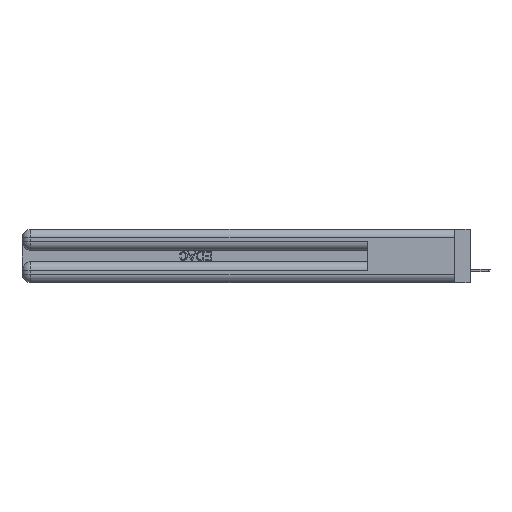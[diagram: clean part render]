
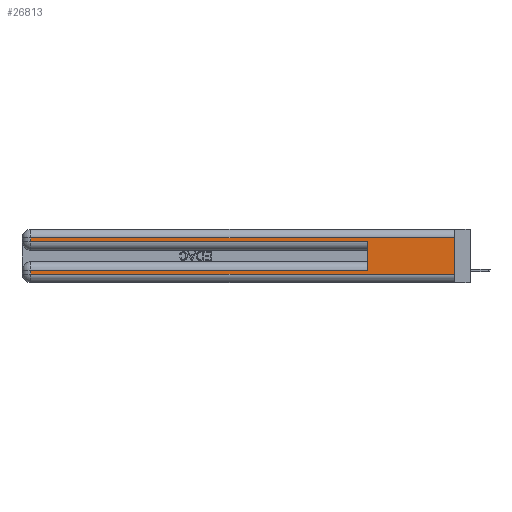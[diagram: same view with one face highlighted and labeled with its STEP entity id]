
A CAD part, left-side view. The second image highlights one B-rep face of the part: STEP entity #26813.
In plain terms, the highlighted planar face has unit normal (-1, 0, 0).
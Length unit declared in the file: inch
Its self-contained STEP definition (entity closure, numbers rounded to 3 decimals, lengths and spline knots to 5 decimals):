
#899 = DIRECTION ( 'NONE',  ( 0., 0., 1. ) ) ;
#1643 = EDGE_CURVE ( 'NONE', #45693, #24644, #16092, .T. ) ;
#1722 = CARTESIAN_POINT ( 'NONE',  ( 0., 0., 0.37 ) ) ;
#3367 = VECTOR ( 'NONE', #18326, 39.37008 ) ;
#3854 = VERTEX_POINT ( 'NONE', #38663 ) ;
#4175 = VECTOR ( 'NONE', #27607, 39.37008 ) ;
#5422 = CARTESIAN_POINT ( 'NONE',  ( 0., 0.6, 0.085 ) ) ;
#5464 = LINE ( 'NONE', #36732, #3367 ) ;
#6622 = ORIENTED_EDGE ( 'NONE', *, *, #1643, .T. ) ;
#7511 = EDGE_CURVE ( 'NONE', #30257, #46423, #32999, .T. ) ;
#7593 = CARTESIAN_POINT ( 'NONE',  ( 0., 0., 0.085 ) ) ;
#7675 = VECTOR ( 'NONE', #27353, 39.37008 ) ;
#7863 = VECTOR ( 'NONE', #13284, 39.37008 ) ;
#7893 = DIRECTION ( 'NONE',  ( 0., -1., 0. ) ) ;
#9753 = ORIENTED_EDGE ( 'NONE', *, *, #15042, .T. ) ;
#11579 = EDGE_CURVE ( 'NONE', #45693, #19201, #28604, .T. ) ;
#12773 = EDGE_LOOP ( 'NONE', ( #22890, #43715, #9753, #49290, #46604, #6622, #43166, #16852 ) ) ;
#13091 = CARTESIAN_POINT ( 'NONE',  ( 0., 0., 0.06 ) ) ;
#13197 = CARTESIAN_POINT ( 'NONE',  ( 0., 2.94, 0.37 ) ) ;
#13284 = DIRECTION ( 'NONE',  ( 0., 0., -1. ) ) ;
#13481 = VERTEX_POINT ( 'NONE', #21888 ) ;
#15042 = EDGE_CURVE ( 'NONE', #24891, #3854, #47481, .T. ) ;
#15576 = LINE ( 'NONE', #31188, #7675 ) ;
#16092 = LINE ( 'NONE', #7593, #4175 ) ;
#16577 = DIRECTION ( 'NONE',  ( 0., 0., -1. ) ) ;
#16852 = ORIENTED_EDGE ( 'NONE', *, *, #35862, .T. ) ;
#18326 = DIRECTION ( 'NONE',  ( 0., 0., -1. ) ) ;
#19201 = VERTEX_POINT ( 'NONE', #46663 ) ;
#19489 = CARTESIAN_POINT ( 'NONE',  ( 0., 0., 0.06 ) ) ;
#19550 = VECTOR ( 'NONE', #899, 39.37008 ) ;
#21888 = CARTESIAN_POINT ( 'NONE',  ( 0., 2.94, 0.06 ) ) ;
#22890 = ORIENTED_EDGE ( 'NONE', *, *, #7511, .F. ) ;
#23029 = EDGE_CURVE ( 'NONE', #3854, #19201, #50371, .T. ) ;
#24139 = DIRECTION ( 'NONE',  ( 0., -1., 0. ) ) ;
#24644 = VERTEX_POINT ( 'NONE', #34574 ) ;
#24891 = VERTEX_POINT ( 'NONE', #37285 ) ;
#26459 = DIRECTION ( 'NONE',  ( 1., 0., 0. ) ) ;
#26609 = EDGE_CURVE ( 'NONE', #30257, #24891, #15576, .T. ) ;
#26702 = CARTESIAN_POINT ( 'NONE',  ( 0., 0., 0.37 ) ) ;
#26813 = ADVANCED_FACE ( 'NONE', ( #30568 ), #42778, .F. ) ;
#26869 = CARTESIAN_POINT ( 'NONE',  ( 0., 0., 0.285 ) ) ;
#27353 = DIRECTION ( 'NONE',  ( 0., 1., 0. ) ) ;
#27607 = DIRECTION ( 'NONE',  ( 0., 1., 0. ) ) ;
#28088 = VECTOR ( 'NONE', #24139, 39.37008 ) ;
#28604 = LINE ( 'NONE', #36000, #19550 ) ;
#30257 = VERTEX_POINT ( 'NONE', #45720 ) ;
#30568 = FACE_OUTER_BOUND ( 'NONE', #12773, .T. ) ;
#31188 = CARTESIAN_POINT ( 'NONE',  ( 0., 0., 0.31 ) ) ;
#32999 = LINE ( 'NONE', #1722, #7863 ) ;
#34262 = EDGE_CURVE ( 'NONE', #24644, #13481, #5464, .T. ) ;
#34574 = CARTESIAN_POINT ( 'NONE',  ( 0., 2.94, 0.085 ) ) ;
#35625 = LINE ( 'NONE', #13091, #28088 ) ;
#35862 = EDGE_CURVE ( 'NONE', #13481, #46423, #35625, .T. ) ;
#36000 = CARTESIAN_POINT ( 'NONE',  ( 0., 0.6, 0.145 ) ) ;
#36316 = AXIS2_PLACEMENT_3D ( 'NONE', #26702, #26459, #50455 ) ;
#36732 = CARTESIAN_POINT ( 'NONE',  ( 0., 2.94, 0.37 ) ) ;
#37285 = CARTESIAN_POINT ( 'NONE',  ( 0., 2.94, 0.31 ) ) ;
#38663 = CARTESIAN_POINT ( 'NONE',  ( 0., 2.94, 0.285 ) ) ;
#42778 = PLANE ( 'NONE',  #36316 ) ;
#43052 = VECTOR ( 'NONE', #16577, 39.37008 ) ;
#43166 = ORIENTED_EDGE ( 'NONE', *, *, #34262, .T. ) ;
#43715 = ORIENTED_EDGE ( 'NONE', *, *, #26609, .T. ) ;
#45693 = VERTEX_POINT ( 'NONE', #5422 ) ;
#45720 = CARTESIAN_POINT ( 'NONE',  ( 0., 0., 0.31 ) ) ;
#46423 = VERTEX_POINT ( 'NONE', #19489 ) ;
#46604 = ORIENTED_EDGE ( 'NONE', *, *, #11579, .F. ) ;
#46663 = CARTESIAN_POINT ( 'NONE',  ( 0., 0.6, 0.285 ) ) ;
#47481 = LINE ( 'NONE', #13197, #43052 ) ;
#49088 = VECTOR ( 'NONE', #7893, 39.37008 ) ;
#49290 = ORIENTED_EDGE ( 'NONE', *, *, #23029, .T. ) ;
#50371 = LINE ( 'NONE', #26869, #49088 ) ;
#50455 = DIRECTION ( 'NONE',  ( 0., 0., -1. ) ) ;
